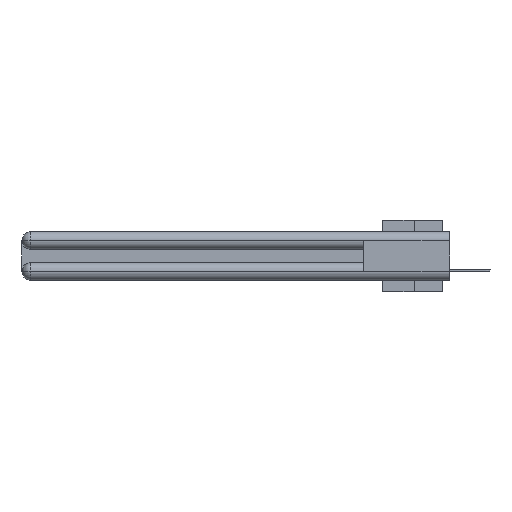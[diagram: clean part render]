
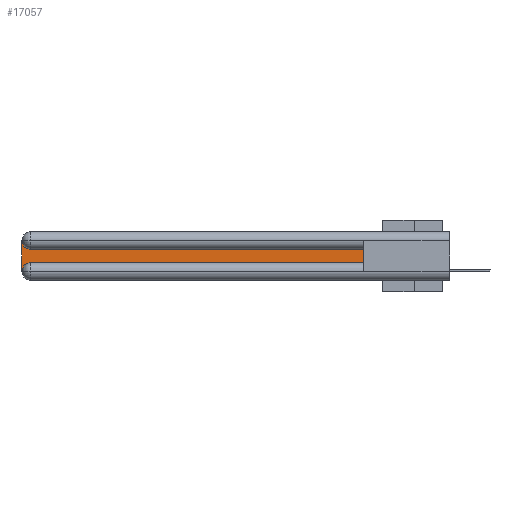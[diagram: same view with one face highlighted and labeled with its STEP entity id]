
A CAD part, left-side view. The second image highlights one B-rep face of the part: STEP entity #17057.
In plain terms, the highlighted planar face has unit normal (-1, 0, 0).
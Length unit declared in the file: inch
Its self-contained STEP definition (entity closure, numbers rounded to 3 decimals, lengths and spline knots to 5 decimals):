
#3917 = PLANE ( 'NONE',  #33498 ) ;
#5851 = EDGE_CURVE ( 'NONE', #18183, #39302, #21399, .T. ) ;
#7219 = VERTEX_POINT ( 'NONE', #16311 ) ;
#7447 = AXIS2_PLACEMENT_3D ( 'NONE', #16934, #16727, #29111 ) ;
#7530 = VERTEX_POINT ( 'NONE', #11834 ) ;
#8004 = EDGE_CURVE ( 'NONE', #17042, #24445, #33706, .T. ) ;
#8223 = DIRECTION ( 'NONE',  ( 0., 0., -1. ) ) ;
#8568 = DIRECTION ( 'NONE',  ( 0., 0., 1. ) ) ;
#9734 = ORIENTED_EDGE ( 'NONE', *, *, #8004, .T. ) ;
#9868 = CARTESIAN_POINT ( 'NONE',  ( 0.075, 2.94, -0.1225 ) ) ;
#10211 = DIRECTION ( 'NONE',  ( 0., 0., -1. ) ) ;
#11294 = CARTESIAN_POINT ( 'NONE',  ( 0.075, 2.94, -0.2775 ) ) ;
#11493 = DIRECTION ( 'NONE',  ( 0., 0., -1. ) ) ;
#11834 = CARTESIAN_POINT ( 'NONE',  ( 0.075, 3., -0.2775 ) ) ;
#12277 = DIRECTION ( 'NONE',  ( 0., -1., 0. ) ) ;
#13633 = EDGE_CURVE ( 'NONE', #24445, #7219, #37899, .T. ) ;
#13803 = CARTESIAN_POINT ( 'NONE',  ( 0.075, 0.6, -0.2175 ) ) ;
#16311 = CARTESIAN_POINT ( 'NONE',  ( 0.075, 3., -0.0625 ) ) ;
#16318 = DIRECTION ( 'NONE',  ( 1., 0., 0. ) ) ;
#16559 = CARTESIAN_POINT ( 'NONE',  ( 0.075, 0.6, -0.2175 ) ) ;
#16727 = DIRECTION ( 'NONE',  ( 1., 0., 0. ) ) ;
#16934 = CARTESIAN_POINT ( 'NONE',  ( 0.075, 2.94, -0.0625 ) ) ;
#17042 = VERTEX_POINT ( 'NONE', #37428 ) ;
#17057 = ADVANCED_FACE ( 'NONE', ( #34591 ), #3917, .F. ) ;
#17285 = ORIENTED_EDGE ( 'NONE', *, *, #5851, .T. ) ;
#18183 = VERTEX_POINT ( 'NONE', #26944 ) ;
#21399 = LINE ( 'NONE', #40051, #25640 ) ;
#22053 = AXIS2_PLACEMENT_3D ( 'NONE', #11294, #33013, #8223 ) ;
#22110 = ORIENTED_EDGE ( 'NONE', *, *, #35463, .T. ) ;
#22429 = VECTOR ( 'NONE', #11493, 39.37008 ) ;
#23075 = CARTESIAN_POINT ( 'NONE',  ( 0.075, 3., -0.2175 ) ) ;
#23468 = LINE ( 'NONE', #23075, #22429 ) ;
#23877 = VECTOR ( 'NONE', #8568, 39.37008 ) ;
#24158 = CARTESIAN_POINT ( 'NONE',  ( 0.075, 0.6, -0.1225 ) ) ;
#24445 = VERTEX_POINT ( 'NONE', #9868 ) ;
#24771 = EDGE_CURVE ( 'NONE', #7530, #18183, #35700, .T. ) ;
#25640 = VECTOR ( 'NONE', #12277, 39.37008 ) ;
#25870 = LINE ( 'NONE', #16559, #23877 ) ;
#26296 = EDGE_LOOP ( 'NONE', ( #9734, #36152, #27816, #33331, #17285, #22110 ) ) ;
#26944 = CARTESIAN_POINT ( 'NONE',  ( 0.075, 2.94, -0.2175 ) ) ;
#27816 = ORIENTED_EDGE ( 'NONE', *, *, #31903, .T. ) ;
#29111 = DIRECTION ( 'NONE',  ( 0., 0., -1. ) ) ;
#31552 = CARTESIAN_POINT ( 'NONE',  ( 0.075, 3., -0.1225 ) ) ;
#31903 = EDGE_CURVE ( 'NONE', #7219, #7530, #23468, .T. ) ;
#33013 = DIRECTION ( 'NONE',  ( 1., 0., 0. ) ) ;
#33331 = ORIENTED_EDGE ( 'NONE', *, *, #24771, .T. ) ;
#33498 = AXIS2_PLACEMENT_3D ( 'NONE', #31552, #16318, #10211 ) ;
#33706 = LINE ( 'NONE', #24158, #35243 ) ;
#34591 = FACE_OUTER_BOUND ( 'NONE', #26296, .T. ) ;
#35243 = VECTOR ( 'NONE', #36550, 39.37008 ) ;
#35463 = EDGE_CURVE ( 'NONE', #39302, #17042, #25870, .T. ) ;
#35700 = CIRCLE ( 'NONE', #22053, 0.06 ) ;
#36152 = ORIENTED_EDGE ( 'NONE', *, *, #13633, .T. ) ;
#36550 = DIRECTION ( 'NONE',  ( 0., 1., 0. ) ) ;
#37428 = CARTESIAN_POINT ( 'NONE',  ( 0.075, 0.6, -0.1225 ) ) ;
#37899 = CIRCLE ( 'NONE', #7447, 0.06 ) ;
#39302 = VERTEX_POINT ( 'NONE', #13803 ) ;
#40051 = CARTESIAN_POINT ( 'NONE',  ( 0.075, 0.6, -0.2175 ) ) ;
